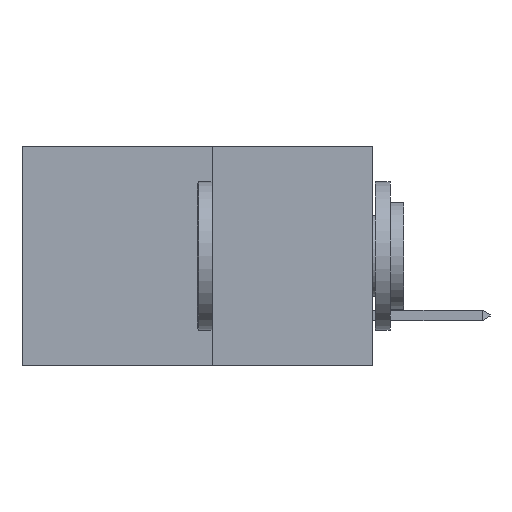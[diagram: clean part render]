
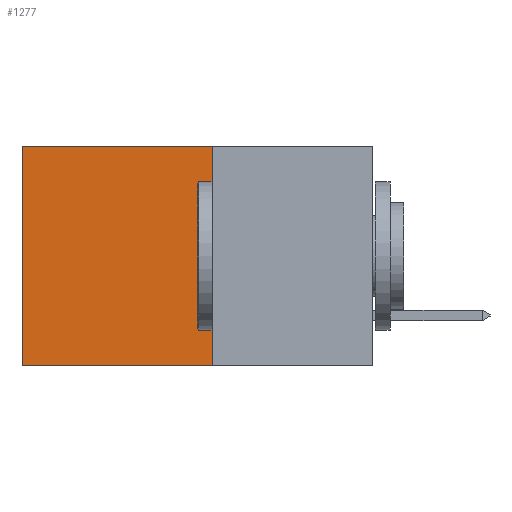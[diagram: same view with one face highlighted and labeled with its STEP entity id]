
A CAD part, left-side view. The second image highlights one B-rep face of the part: STEP entity #1277.
In plain terms, the highlighted planar face has unit normal (-1, 0, 0).
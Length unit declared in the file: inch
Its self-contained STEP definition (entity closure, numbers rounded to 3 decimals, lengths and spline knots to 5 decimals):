
#30 = CARTESIAN_POINT ( 'NONE',  ( 0.277, 0.59, 0. ) ) ;
#619 = EDGE_CURVE ( 'NONE', #4934, #1843, #1475, .T. ) ;
#1277 = ADVANCED_FACE ( 'NONE', ( #6567 ), #3363, .F. ) ;
#1393 = VERTEX_POINT ( 'NONE', #11830 ) ;
#1475 = LINE ( 'NONE', #7707, #6431 ) ;
#1612 = DIRECTION ( 'NONE',  ( 0., 0., -1. ) ) ;
#1635 = EDGE_CURVE ( 'NONE', #2353, #4934, #2517, .T. ) ;
#1843 = VERTEX_POINT ( 'NONE', #2049 ) ;
#1852 = VECTOR ( 'NONE', #9784, 39.37008 ) ;
#2049 = CARTESIAN_POINT ( 'NONE',  ( 0.277, 0.59, -0.37 ) ) ;
#2161 = LINE ( 'NONE', #10774, #1852 ) ;
#2353 = VERTEX_POINT ( 'NONE', #2644 ) ;
#2517 = LINE ( 'NONE', #7048, #3128 ) ;
#2644 = CARTESIAN_POINT ( 'NONE',  ( 0.277, 0.27, 0. ) ) ;
#3128 = VECTOR ( 'NONE', #7892, 39.37008 ) ;
#3319 = DIRECTION ( 'NONE',  ( 0., 0., -1. ) ) ;
#3322 = CARTESIAN_POINT ( 'NONE',  ( 0.277, 0.27, -0.37 ) ) ;
#3363 = PLANE ( 'NONE',  #6319 ) ;
#3556 = LINE ( 'NONE', #6169, #8482 ) ;
#4934 = VERTEX_POINT ( 'NONE', #30 ) ;
#5116 = ORIENTED_EDGE ( 'NONE', *, *, #619, .T. ) ;
#5143 = ORIENTED_EDGE ( 'NONE', *, *, #6351, .F. ) ;
#5155 = ORIENTED_EDGE ( 'NONE', *, *, #5487, .F. ) ;
#5203 = ORIENTED_EDGE ( 'NONE', *, *, #1635, .T. ) ;
#5487 = EDGE_CURVE ( 'NONE', #2353, #1393, #3556, .T. ) ;
#6169 = CARTESIAN_POINT ( 'NONE',  ( 0.277, 0.27, -0.37 ) ) ;
#6313 = DIRECTION ( 'NONE',  ( 0., 0., -1. ) ) ;
#6319 = AXIS2_PLACEMENT_3D ( 'NONE', #3322, #10560, #3319 ) ;
#6351 = EDGE_CURVE ( 'NONE', #1393, #1843, #2161, .T. ) ;
#6431 = VECTOR ( 'NONE', #1612, 39.37008 ) ;
#6567 = FACE_OUTER_BOUND ( 'NONE', #10616, .T. ) ;
#7048 = CARTESIAN_POINT ( 'NONE',  ( 0.277, 0.27, 0. ) ) ;
#7707 = CARTESIAN_POINT ( 'NONE',  ( 0.277, 0.59, -0.37 ) ) ;
#7892 = DIRECTION ( 'NONE',  ( 0., 1., 0. ) ) ;
#8482 = VECTOR ( 'NONE', #6313, 39.37008 ) ;
#9784 = DIRECTION ( 'NONE',  ( 0., 1., 0. ) ) ;
#10560 = DIRECTION ( 'NONE',  ( 1., 0., 0. ) ) ;
#10616 = EDGE_LOOP ( 'NONE', ( #5116, #5143, #5155, #5203 ) ) ;
#10774 = CARTESIAN_POINT ( 'NONE',  ( 0.277, 0.27, -0.37 ) ) ;
#11830 = CARTESIAN_POINT ( 'NONE',  ( 0.277, 0.27, -0.37 ) ) ;
